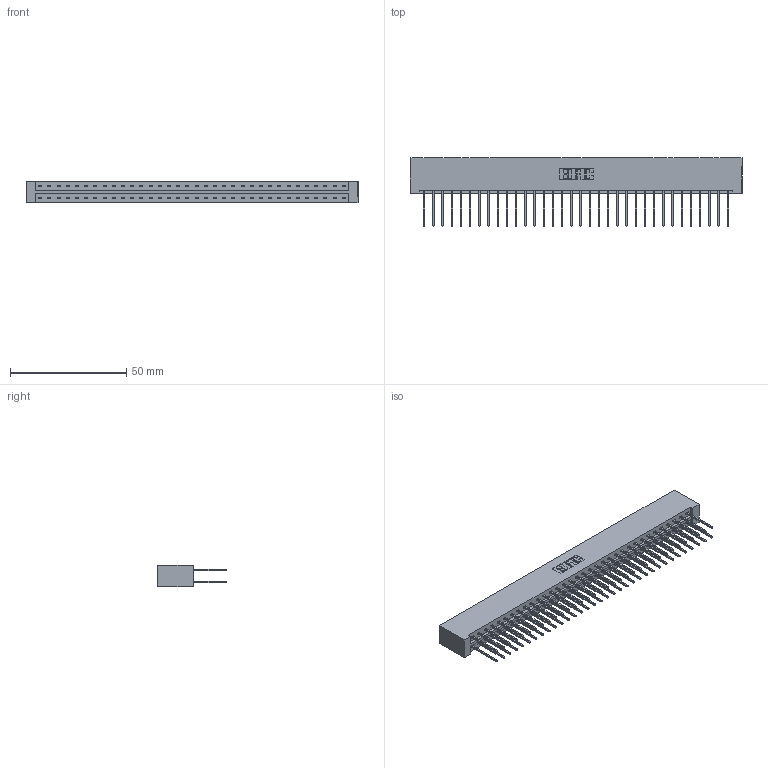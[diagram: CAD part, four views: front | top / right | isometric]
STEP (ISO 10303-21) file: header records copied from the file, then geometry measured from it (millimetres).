
FILE_DESCRIPTION (( 'STEP AP203' ), '1' );
FILE_NAME ('833-068-540-201.STEP', '2020-06-05T10:32:40', ( '' ), ( '' ), 'SwSTEP 2.0', 'SolidWorks 2020', '' );
FILE_SCHEMA (( 'CONFIG_CONTROL_DESIGN' ));
Length unit declared in the file: inch
Products named in the file (3): 833-068-540-201; 833 Part_Lugless; 345-292-001_345-293-140
Assembly tree (69 placements, depth 2):
  833-068-540-201
    833 Part_Lugless
    345-292-001_345-293-140  x68
Bounding box: 142.98 x 29.47 x 9.4 mm (x, y, z)
Volume: 15412.3 mm3; surface area: 19425.1 mm2
Topology: 69 solids, 69 shells, 3642 faces, 10827 edges, 7126 vertices
Faces by surface type: plane 2514, cylinder 1128
Entity records: 22649 total; most frequent: CARTESIAN_POINT 3762, ORIENTED_EDGE 3698, DIRECTION 3221, EDGE_CURVE 1849, VECTOR 1729, LINE 1729, VERTEX_POINT 1230, AXIS2_PLACEMENT_3D 746
